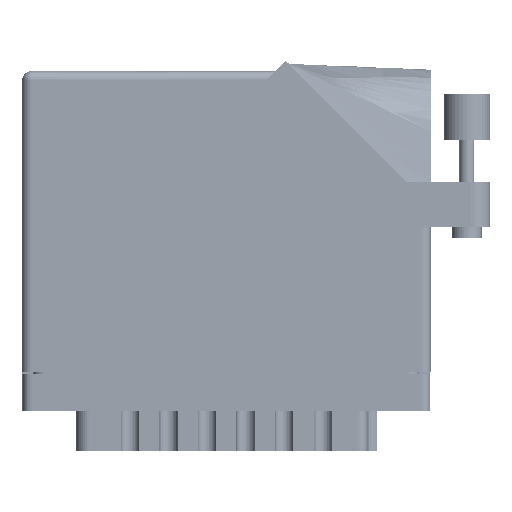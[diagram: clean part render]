
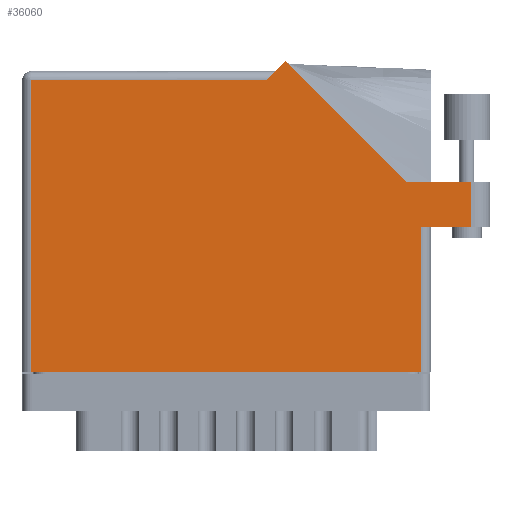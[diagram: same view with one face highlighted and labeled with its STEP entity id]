
A CAD part, front view. The second image highlights one B-rep face of the part: STEP entity #36060.
In plain terms, the highlighted face is planar.
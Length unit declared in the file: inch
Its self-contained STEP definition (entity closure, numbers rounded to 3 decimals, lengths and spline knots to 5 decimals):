
#3711 = DIRECTION ( 'NONE',  ( -1., 0., 0. ) ) ;
#5505 = EDGE_CURVE ( 'NONE', #51776, #89199, #54160, .T. ) ;
#7237 = EDGE_LOOP ( 'NONE', ( #94878, #75354, #8061, #10782, #31484, #85595, #40029, #40410, #61153 ) ) ;
#8061 = ORIENTED_EDGE ( 'NONE', *, *, #23873, .T. ) ;
#10175 = DIRECTION ( 'NONE',  ( -0.707, 0.707, 0. ) ) ;
#10782 = ORIENTED_EDGE ( 'NONE', *, *, #46216, .T. ) ;
#12212 = EDGE_CURVE ( 'NONE', #89199, #46669, #92869, .T. ) ;
#12352 = LINE ( 'NONE', #90654, #74052 ) ;
#12583 = VERTEX_POINT ( 'NONE', #59749 ) ;
#13897 = DIRECTION ( 'NONE',  ( 0., 1., 0. ) ) ;
#18099 = CARTESIAN_POINT ( 'NONE',  ( 0., 2.03, 0. ) ) ;
#23390 = VERTEX_POINT ( 'NONE', #94361 ) ;
#23873 = EDGE_CURVE ( 'NONE', #46669, #88564, #53207, .T. ) ;
#26862 = VERTEX_POINT ( 'NONE', #40407 ) ;
#28968 = EDGE_CURVE ( 'NONE', #23390, #48110, #70764, .T. ) ;
#29571 = CARTESIAN_POINT ( 'NONE',  ( 3.03, 1.287, 0. ) ) ;
#30502 = EDGE_CURVE ( 'NONE', #48110, #26862, #12352, .T. ) ;
#31484 = ORIENTED_EDGE ( 'NONE', *, *, #28968, .T. ) ;
#34008 = DIRECTION ( 'NONE',  ( 0., -1., 0. ) ) ;
#34558 = CARTESIAN_POINT ( 'NONE',  ( 3.155, 1.287, 0. ) ) ;
#36060 = ADVANCED_FACE ( 'NONE', ( #82297 ), #48064, .F. ) ;
#36958 = CARTESIAN_POINT ( 'NONE',  ( 1.705, 2.03, 0. ) ) ;
#38132 = DIRECTION ( 'NONE',  ( 1., 0., 0. ) ) ;
#39980 = DIRECTION ( 'NONE',  ( 0., 1., 0. ) ) ;
#40029 = ORIENTED_EDGE ( 'NONE', *, *, #85055, .T. ) ;
#40407 = CARTESIAN_POINT ( 'NONE',  ( 0.062, 1.968, 0. ) ) ;
#40410 = ORIENTED_EDGE ( 'NONE', *, *, #67642, .T. ) ;
#40558 = CARTESIAN_POINT ( 'NONE',  ( 3.03, 0.98, 0. ) ) ;
#40891 = CARTESIAN_POINT ( 'NONE',  ( 2.755, 0.98, 0. ) ) ;
#42475 = VECTOR ( 'NONE', #64661, 39.37008 ) ;
#44790 = DIRECTION ( 'NONE',  ( -0.707, -0.707, 0. ) ) ;
#46216 = EDGE_CURVE ( 'NONE', #88564, #23390, #92217, .T. ) ;
#46669 = VERTEX_POINT ( 'NONE', #29571 ) ;
#46677 = VECTOR ( 'NONE', #10175, 39.37008 ) ;
#48064 = PLANE ( 'NONE',  #73044 ) ;
#48110 = VERTEX_POINT ( 'NONE', #79890 ) ;
#48663 = VECTOR ( 'NONE', #44790, 39.37008 ) ;
#51776 = VERTEX_POINT ( 'NONE', #66591 ) ;
#51874 = LINE ( 'NONE', #57866, #67022 ) ;
#53207 = LINE ( 'NONE', #34558, #78792 ) ;
#54160 = LINE ( 'NONE', #40891, #42475 ) ;
#54917 = DIRECTION ( 'NONE',  ( 0., 0., -1. ) ) ;
#55348 = VECTOR ( 'NONE', #34008, 39.37008 ) ;
#57866 = CARTESIAN_POINT ( 'NONE',  ( 2.693, 0.98, 0. ) ) ;
#58318 = CARTESIAN_POINT ( 'NONE',  ( 2.693, 0., 0. ) ) ;
#59749 = CARTESIAN_POINT ( 'NONE',  ( 0.062, 0., 0. ) ) ;
#61153 = ORIENTED_EDGE ( 'NONE', *, *, #63839, .T. ) ;
#62811 = CARTESIAN_POINT ( 'NONE',  ( 2.58942, 1.287, 0. ) ) ;
#63032 = DIRECTION ( 'NONE',  ( -1., 0., 0. ) ) ;
#63839 = EDGE_CURVE ( 'NONE', #72990, #51776, #51874, .T. ) ;
#64661 = DIRECTION ( 'NONE',  ( 1., 0., 0. ) ) ;
#66591 = CARTESIAN_POINT ( 'NONE',  ( 2.693, 0.98, 0. ) ) ;
#67022 = VECTOR ( 'NONE', #13897, 39.37008 ) ;
#67642 = EDGE_CURVE ( 'NONE', #12583, #72990, #71054, .T. ) ;
#68737 = VECTOR ( 'NONE', #38132, 39.37008 ) ;
#70764 = LINE ( 'NONE', #36958, #48663 ) ;
#71054 = LINE ( 'NONE', #82392, #68737 ) ;
#72990 = VERTEX_POINT ( 'NONE', #58318 ) ;
#73044 = AXIS2_PLACEMENT_3D ( 'NONE', #18099, #54917, #63032 ) ;
#74052 = VECTOR ( 'NONE', #75936, 39.37008 ) ;
#75354 = ORIENTED_EDGE ( 'NONE', *, *, #12212, .T. ) ;
#75936 = DIRECTION ( 'NONE',  ( -1., 0., 0. ) ) ;
#76572 = CARTESIAN_POINT ( 'NONE',  ( 2.58942, 1.287, 0. ) ) ;
#78792 = VECTOR ( 'NONE', #3711, 39.37008 ) ;
#79890 = CARTESIAN_POINT ( 'NONE',  ( 1.643, 1.968, 0. ) ) ;
#79997 = VECTOR ( 'NONE', #39980, 39.37008 ) ;
#82297 = FACE_OUTER_BOUND ( 'NONE', #7237, .T. ) ;
#82392 = CARTESIAN_POINT ( 'NONE',  ( 0., 0., 0. ) ) ;
#83264 = CARTESIAN_POINT ( 'NONE',  ( 3.03, 1.287, 0. ) ) ;
#85055 = EDGE_CURVE ( 'NONE', #26862, #12583, #93896, .T. ) ;
#85595 = ORIENTED_EDGE ( 'NONE', *, *, #30502, .T. ) ;
#88564 = VERTEX_POINT ( 'NONE', #62811 ) ;
#89199 = VERTEX_POINT ( 'NONE', #40558 ) ;
#90654 = CARTESIAN_POINT ( 'NONE',  ( 0., 1.968, 0. ) ) ;
#92217 = LINE ( 'NONE', #76572, #46677 ) ;
#92869 = LINE ( 'NONE', #83264, #79997 ) ;
#93035 = CARTESIAN_POINT ( 'NONE',  ( 0.062, 0., 0. ) ) ;
#93896 = LINE ( 'NONE', #93035, #55348 ) ;
#94361 = CARTESIAN_POINT ( 'NONE',  ( 1.77571, 2.10071, 0. ) ) ;
#94878 = ORIENTED_EDGE ( 'NONE', *, *, #5505, .T. ) ;
